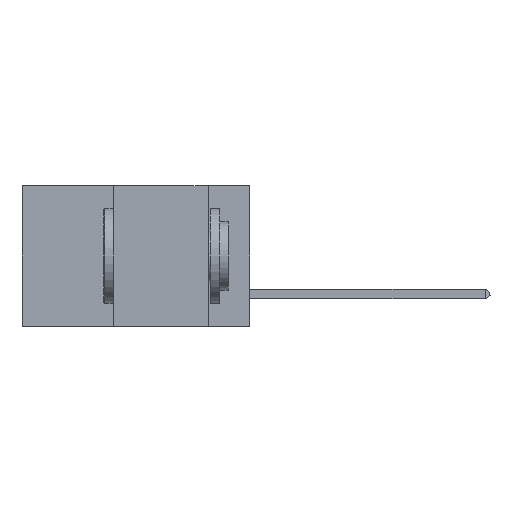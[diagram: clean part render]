
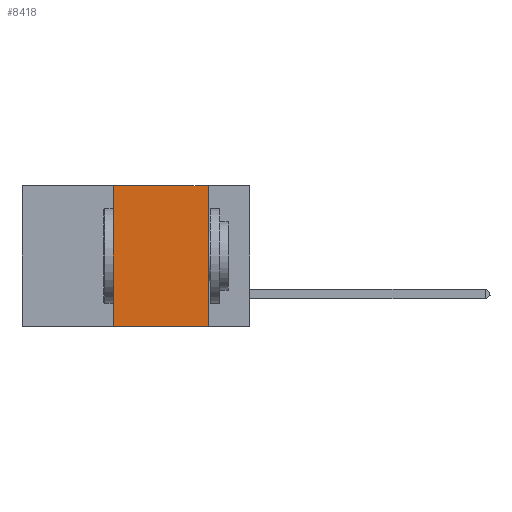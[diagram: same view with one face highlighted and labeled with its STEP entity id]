
A CAD part, left-side view. The second image highlights one B-rep face of the part: STEP entity #8418.
In plain terms, the highlighted planar face has unit normal (-1, 0, 0).
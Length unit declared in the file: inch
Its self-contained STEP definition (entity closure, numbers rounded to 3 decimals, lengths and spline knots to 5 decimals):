
#94 = DIRECTION ( 'NONE',  ( 1., 0., 0. ) ) ;
#668 = ORIENTED_EDGE ( 'NONE', *, *, #9830, .F. ) ;
#985 = LINE ( 'NONE', #10710, #8636 ) ;
#987 = DIRECTION ( 'NONE',  ( 0., 0., -1. ) ) ;
#1584 = LINE ( 'NONE', #5923, #3649 ) ;
#2408 = EDGE_LOOP ( 'NONE', ( #668, #6594, #6806, #3117 ) ) ;
#3117 = ORIENTED_EDGE ( 'NONE', *, *, #5925, .T. ) ;
#3649 = VECTOR ( 'NONE', #987, 39.37008 ) ;
#3878 = LINE ( 'NONE', #8423, #4527 ) ;
#4368 = CARTESIAN_POINT ( 'NONE',  ( 0., 0.11, 0. ) ) ;
#4527 = VECTOR ( 'NONE', #8277, 39.37008 ) ;
#4674 = DIRECTION ( 'NONE',  ( 0., -1., 0. ) ) ;
#4893 = LINE ( 'NONE', #6297, #6300 ) ;
#5047 = CARTESIAN_POINT ( 'NONE',  ( 0., 0.6, 0. ) ) ;
#5708 = CARTESIAN_POINT ( 'NONE',  ( 0., 0.36, 0. ) ) ;
#5923 = CARTESIAN_POINT ( 'NONE',  ( 0., 0.11, 0. ) ) ;
#5925 = EDGE_CURVE ( 'NONE', #8178, #9303, #3878, .T. ) ;
#6149 = FACE_OUTER_BOUND ( 'NONE', #2408, .T. ) ;
#6297 = CARTESIAN_POINT ( 'NONE',  ( 0., 0.6, 0. ) ) ;
#6300 = VECTOR ( 'NONE', #4674, 39.37008 ) ;
#6594 = ORIENTED_EDGE ( 'NONE', *, *, #7443, .F. ) ;
#6806 = ORIENTED_EDGE ( 'NONE', *, *, #7749, .F. ) ;
#6954 = CARTESIAN_POINT ( 'NONE',  ( 0., 0.11, -0.37 ) ) ;
#7006 = CARTESIAN_POINT ( 'NONE',  ( 0., 0.36, -0.37 ) ) ;
#7278 = DIRECTION ( 'NONE',  ( 0., 0., 1. ) ) ;
#7443 = EDGE_CURVE ( 'NONE', #10454, #9885, #4893, .T. ) ;
#7492 = PLANE ( 'NONE',  #10331 ) ;
#7749 = EDGE_CURVE ( 'NONE', #8178, #10454, #985, .T. ) ;
#8178 = VERTEX_POINT ( 'NONE', #7006 ) ;
#8277 = DIRECTION ( 'NONE',  ( 0., -1., 0. ) ) ;
#8418 = ADVANCED_FACE ( 'NONE', ( #6149 ), #7492, .F. ) ;
#8423 = CARTESIAN_POINT ( 'NONE',  ( 0., 0.6, -0.37 ) ) ;
#8636 = VECTOR ( 'NONE', #7278, 39.37008 ) ;
#9303 = VERTEX_POINT ( 'NONE', #6954 ) ;
#9830 = EDGE_CURVE ( 'NONE', #9885, #9303, #1584, .T. ) ;
#9885 = VERTEX_POINT ( 'NONE', #4368 ) ;
#10009 = DIRECTION ( 'NONE',  ( 0., 0., -1. ) ) ;
#10331 = AXIS2_PLACEMENT_3D ( 'NONE', #5047, #94, #10009 ) ;
#10454 = VERTEX_POINT ( 'NONE', #5708 ) ;
#10710 = CARTESIAN_POINT ( 'NONE',  ( 0., 0.36, 0. ) ) ;
